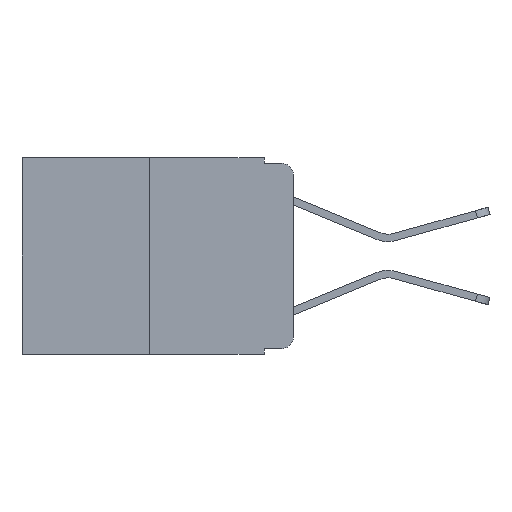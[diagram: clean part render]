
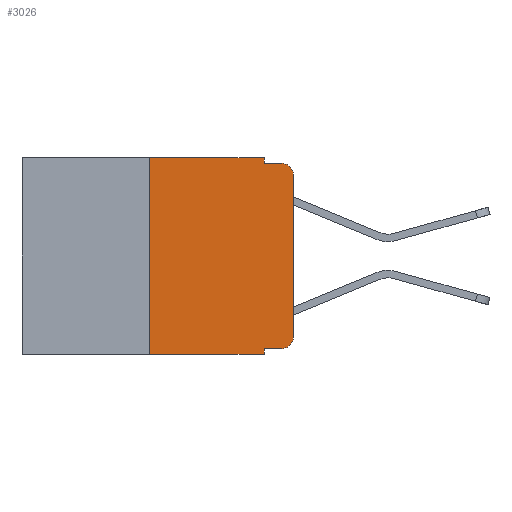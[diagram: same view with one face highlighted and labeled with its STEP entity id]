
A CAD part, left-side view. The second image highlights one B-rep face of the part: STEP entity #3026.
In plain terms, the highlighted planar face has unit normal (-1, 0, 0).
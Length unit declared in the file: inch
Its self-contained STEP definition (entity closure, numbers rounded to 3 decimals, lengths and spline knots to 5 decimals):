
#423 = DIRECTION ( 'NONE',  ( 0., 0., -1. ) ) ;
#428 = CARTESIAN_POINT ( 'NONE',  ( 0., 0.051, -0.01 ) ) ;
#1151 = FACE_OUTER_BOUND ( 'NONE', #4532, .T. ) ;
#1337 = EDGE_CURVE ( 'NONE', #3234, #2053, #14423, .T. ) ;
#1565 = VECTOR ( 'NONE', #12152, 39.37008 ) ;
#2053 = VERTEX_POINT ( 'NONE', #10339 ) ;
#2212 = LINE ( 'NONE', #12283, #14048 ) ;
#2229 = VECTOR ( 'NONE', #10138, 39.37008 ) ;
#2307 = DIRECTION ( 'NONE',  ( -1., 0., 0. ) ) ;
#2556 = LINE ( 'NONE', #5118, #8215 ) ;
#2895 = ORIENTED_EDGE ( 'NONE', *, *, #4292, .T. ) ;
#2967 = ORIENTED_EDGE ( 'NONE', *, *, #12447, .T. ) ;
#3026 = ADVANCED_FACE ( 'NONE', ( #1151 ), #5051, .F. ) ;
#3129 = ORIENTED_EDGE ( 'NONE', *, *, #11746, .F. ) ;
#3234 = VERTEX_POINT ( 'NONE', #9821 ) ;
#3287 = ORIENTED_EDGE ( 'NONE', *, *, #8017, .F. ) ;
#3325 = ORIENTED_EDGE ( 'NONE', *, *, #10824, .T. ) ;
#3401 = EDGE_CURVE ( 'NONE', #8241, #8412, #2212, .T. ) ;
#3420 = LINE ( 'NONE', #3605, #6105 ) ;
#3427 = AXIS2_PLACEMENT_3D ( 'NONE', #5303, #6967, #11524 ) ;
#3508 = ORIENTED_EDGE ( 'NONE', *, *, #6566, .F. ) ;
#3605 = CARTESIAN_POINT ( 'NONE',  ( 0., 0.051, 0. ) ) ;
#3750 = CARTESIAN_POINT ( 'NONE',  ( 0., 0.02, -0.01 ) ) ;
#3816 = ORIENTED_EDGE ( 'NONE', *, *, #3401, .F. ) ;
#3905 = ORIENTED_EDGE ( 'NONE', *, *, #5785, .F. ) ;
#4155 = ORIENTED_EDGE ( 'NONE', *, *, #5061, .T. ) ;
#4282 = CARTESIAN_POINT ( 'NONE',  ( 0., 0.051, -0.343 ) ) ;
#4292 = EDGE_CURVE ( 'NONE', #2053, #12557, #2556, .T. ) ;
#4303 = CARTESIAN_POINT ( 'NONE',  ( 0., 0.051, 0. ) ) ;
#4532 = EDGE_LOOP ( 'NONE', ( #2895, #4155, #3905, #3508, #3816, #3287, #3325, #3129, #2967, #5564 ) ) ;
#5023 = CARTESIAN_POINT ( 'NONE',  ( 0., 0.051, 0. ) ) ;
#5051 = PLANE ( 'NONE',  #9596 ) ;
#5061 = EDGE_CURVE ( 'NONE', #12557, #10894, #12846, .T. ) ;
#5118 = CARTESIAN_POINT ( 'NONE',  ( 0., 0., 0. ) ) ;
#5303 = CARTESIAN_POINT ( 'NONE',  ( 0., 0.02, -0.313 ) ) ;
#5564 = ORIENTED_EDGE ( 'NONE', *, *, #1337, .T. ) ;
#5785 = EDGE_CURVE ( 'NONE', #8954, #10894, #13181, .T. ) ;
#5894 = DIRECTION ( 'NONE',  ( 0., -1., 0. ) ) ;
#6105 = VECTOR ( 'NONE', #10336, 39.37008 ) ;
#6566 = EDGE_CURVE ( 'NONE', #8412, #8954, #3420, .T. ) ;
#6967 = DIRECTION ( 'NONE',  ( -1., 0., 0. ) ) ;
#7103 = LINE ( 'NONE', #10372, #12271 ) ;
#7288 = DIRECTION ( 'NONE',  ( 1., 0., 0. ) ) ;
#8017 = EDGE_CURVE ( 'NONE', #10484, #8241, #10241, .T. ) ;
#8069 = CARTESIAN_POINT ( 'NONE',  ( 0., 0., -0.03 ) ) ;
#8215 = VECTOR ( 'NONE', #13882, 39.37008 ) ;
#8241 = VERTEX_POINT ( 'NONE', #9228 ) ;
#8412 = VERTEX_POINT ( 'NONE', #5023 ) ;
#8954 = VERTEX_POINT ( 'NONE', #9447 ) ;
#9113 = CARTESIAN_POINT ( 'NONE',  ( 0., 0.02, -0.03 ) ) ;
#9228 = CARTESIAN_POINT ( 'NONE',  ( 0., 0.25, 0. ) ) ;
#9447 = CARTESIAN_POINT ( 'NONE',  ( 0., 0.051, -0.01 ) ) ;
#9596 = AXIS2_PLACEMENT_3D ( 'NONE', #13814, #7288, #423 ) ;
#9671 = CARTESIAN_POINT ( 'NONE',  ( 0., 0.25, -0.343 ) ) ;
#9821 = CARTESIAN_POINT ( 'NONE',  ( 0., 0.02, -0.333 ) ) ;
#10138 = DIRECTION ( 'NONE',  ( 0., -1., 0. ) ) ;
#10217 = DIRECTION ( 'NONE',  ( 0., 0., -1. ) ) ;
#10241 = LINE ( 'NONE', #11061, #1565 ) ;
#10303 = VECTOR ( 'NONE', #11739, 39.37008 ) ;
#10336 = DIRECTION ( 'NONE',  ( 0., 0., -1. ) ) ;
#10339 = CARTESIAN_POINT ( 'NONE',  ( 0., 0., -0.313 ) ) ;
#10372 = CARTESIAN_POINT ( 'NONE',  ( 0., 0.473, -0.343 ) ) ;
#10484 = VERTEX_POINT ( 'NONE', #9671 ) ;
#10605 = VERTEX_POINT ( 'NONE', #4282 ) ;
#10824 = EDGE_CURVE ( 'NONE', #10484, #10605, #7103, .T. ) ;
#10853 = VERTEX_POINT ( 'NONE', #12599 ) ;
#10892 = LINE ( 'NONE', #14389, #2229 ) ;
#10894 = VERTEX_POINT ( 'NONE', #3750 ) ;
#10982 = DIRECTION ( 'NONE',  ( 0., 0., -1. ) ) ;
#11061 = CARTESIAN_POINT ( 'NONE',  ( 0., 0.25, 0. ) ) ;
#11417 = VECTOR ( 'NONE', #10982, 39.37008 ) ;
#11524 = DIRECTION ( 'NONE',  ( 0., 0., -1. ) ) ;
#11739 = DIRECTION ( 'NONE',  ( 0., -1., 0. ) ) ;
#11746 = EDGE_CURVE ( 'NONE', #10853, #10605, #14246, .T. ) ;
#12152 = DIRECTION ( 'NONE',  ( 0., 0., 1. ) ) ;
#12271 = VECTOR ( 'NONE', #5894, 39.37008 ) ;
#12283 = CARTESIAN_POINT ( 'NONE',  ( 0., 0.473, 0. ) ) ;
#12447 = EDGE_CURVE ( 'NONE', #10853, #3234, #10892, .T. ) ;
#12557 = VERTEX_POINT ( 'NONE', #8069 ) ;
#12599 = CARTESIAN_POINT ( 'NONE',  ( 0., 0.051, -0.333 ) ) ;
#12846 = CIRCLE ( 'NONE', #14447, 0.02 ) ;
#13181 = LINE ( 'NONE', #428, #10303 ) ;
#13302 = DIRECTION ( 'NONE',  ( 0., -1., 0. ) ) ;
#13814 = CARTESIAN_POINT ( 'NONE',  ( 0., 0.473, 0. ) ) ;
#13882 = DIRECTION ( 'NONE',  ( 0., 0., 1. ) ) ;
#14048 = VECTOR ( 'NONE', #13302, 39.37008 ) ;
#14246 = LINE ( 'NONE', #4303, #11417 ) ;
#14389 = CARTESIAN_POINT ( 'NONE',  ( 0., 0.051, -0.333 ) ) ;
#14423 = CIRCLE ( 'NONE', #3427, 0.02 ) ;
#14447 = AXIS2_PLACEMENT_3D ( 'NONE', #9113, #2307, #10217 ) ;
